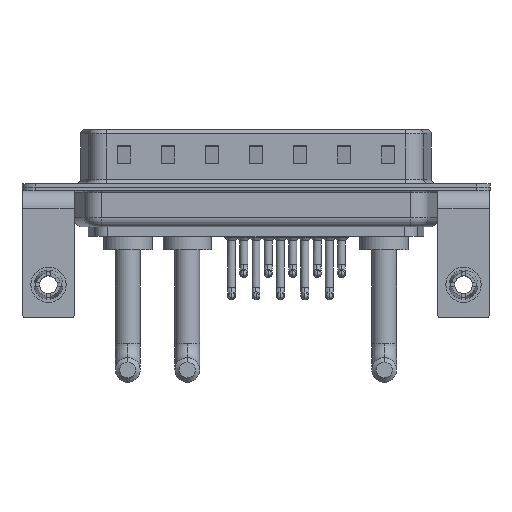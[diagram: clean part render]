
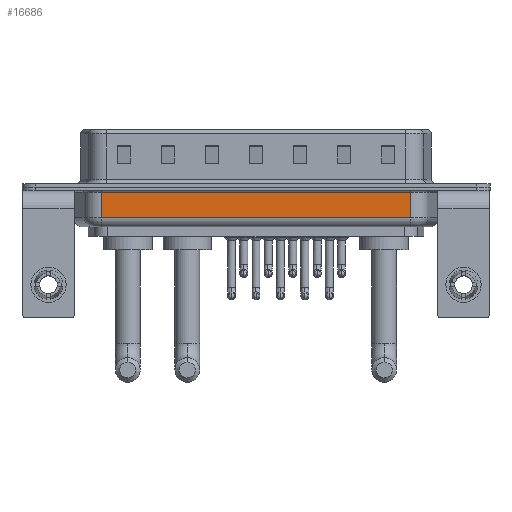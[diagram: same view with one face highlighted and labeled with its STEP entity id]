
A CAD part, front view. The second image highlights one B-rep face of the part: STEP entity #16686.
In plain terms, the highlighted planar face has unit normal (0, -1, 0).
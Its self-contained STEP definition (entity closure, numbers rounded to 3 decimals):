
#351 = CARTESIAN_POINT ( 'NONE',  ( 6.006, -5.35, -4.5 ) ) ;
#1069 = ORIENTED_EDGE ( 'NONE', *, *, #25757, .T. ) ;
#1312 = CARTESIAN_POINT ( 'NONE',  ( 41.044, -5.35, -0.65 ) ) ;
#1676 = CARTESIAN_POINT ( 'NONE',  ( 6.006, -5.35, -3.5 ) ) ;
#2877 = ORIENTED_EDGE ( 'NONE', *, *, #8427, .T. ) ;
#3268 = VECTOR ( 'NONE', #16015, 1000. ) ;
#3957 = DIRECTION ( 'NONE',  ( 0., 1., 0. ) ) ;
#5058 = CARTESIAN_POINT ( 'NONE',  ( 41.044, -5.35, -4.5 ) ) ;
#6736 = DIRECTION ( 'NONE',  ( 1., 0., 0. ) ) ;
#7129 = LINE ( 'NONE', #10952, #11258 ) ;
#8283 = LINE ( 'NONE', #351, #22655 ) ;
#8427 = EDGE_CURVE ( 'NONE', #23445, #17017, #10984, .T. ) ;
#9786 = CARTESIAN_POINT ( 'NONE',  ( 41.044, -5.35, -3.5 ) ) ;
#10273 = AXIS2_PLACEMENT_3D ( 'NONE', #25812, #3957, #16028 ) ;
#10952 = CARTESIAN_POINT ( 'NONE',  ( 6.006, -5.35, -3.5 ) ) ;
#10983 = LINE ( 'NONE', #23678, #3268 ) ;
#10984 = LINE ( 'NONE', #5058, #15872 ) ;
#11258 = VECTOR ( 'NONE', #6736, 1000. ) ;
#11453 = EDGE_LOOP ( 'NONE', ( #18125, #1069, #2877, #21312 ) ) ;
#14012 = FACE_OUTER_BOUND ( 'NONE', #11453, .T. ) ;
#15872 = VECTOR ( 'NONE', #16704, 1000. ) ;
#16015 = DIRECTION ( 'NONE',  ( -1., 0., 0. ) ) ;
#16028 = DIRECTION ( 'NONE',  ( 0., 0., 1. ) ) ;
#16686 = ADVANCED_FACE ( 'NONE', ( #14012 ), #26075, .F. ) ;
#16704 = DIRECTION ( 'NONE',  ( 0., 0., 1. ) ) ;
#17017 = VERTEX_POINT ( 'NONE', #1312 ) ;
#18125 = ORIENTED_EDGE ( 'NONE', *, *, #19079, .F. ) ;
#18928 = VERTEX_POINT ( 'NONE', #1676 ) ;
#19079 = EDGE_CURVE ( 'NONE', #18928, #20404, #8283, .T. ) ;
#19945 = EDGE_CURVE ( 'NONE', #17017, #20404, #10983, .T. ) ;
#20404 = VERTEX_POINT ( 'NONE', #21141 ) ;
#21141 = CARTESIAN_POINT ( 'NONE',  ( 6.006, -5.35, -0.65 ) ) ;
#21312 = ORIENTED_EDGE ( 'NONE', *, *, #19945, .T. ) ;
#22655 = VECTOR ( 'NONE', #24280, 1000. ) ;
#23445 = VERTEX_POINT ( 'NONE', #9786 ) ;
#23678 = CARTESIAN_POINT ( 'NONE',  ( 6.006, -5.35, -0.65 ) ) ;
#24280 = DIRECTION ( 'NONE',  ( 0., 0., 1. ) ) ;
#25757 = EDGE_CURVE ( 'NONE', #18928, #23445, #7129, .T. ) ;
#25812 = CARTESIAN_POINT ( 'NONE',  ( 6.006, -5.35, -4.5 ) ) ;
#26075 = PLANE ( 'NONE',  #10273 ) ;
